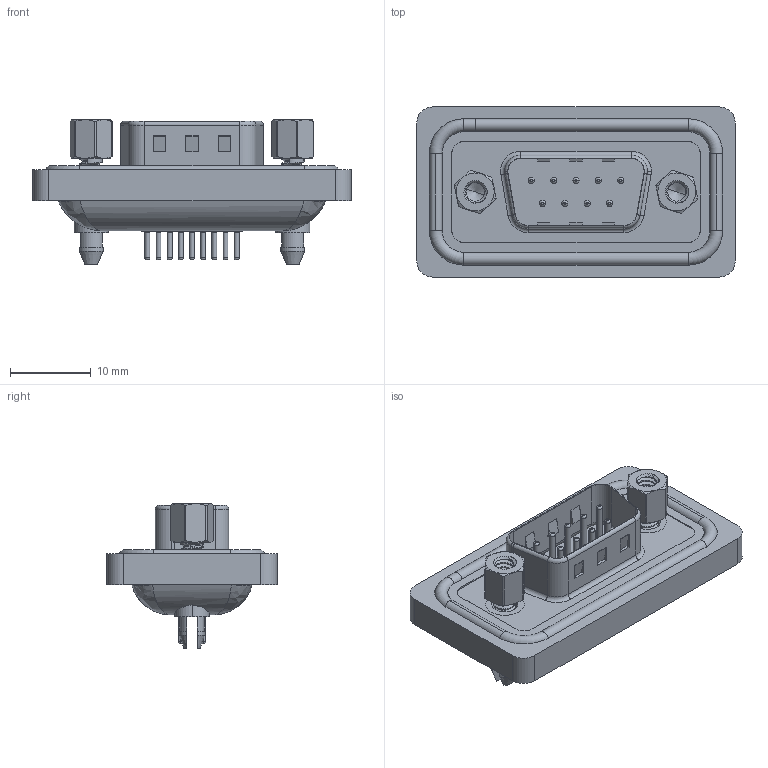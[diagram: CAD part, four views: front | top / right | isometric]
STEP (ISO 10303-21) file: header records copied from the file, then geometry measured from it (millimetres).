
FILE_DESCRIPTION (( 'STEP AP203' ), '1' );
FILE_NAME ('627-W09-320-013.STEP', '2024-03-19T11:55:11', ( '' ), ( '' ), 'SwSTEP 2.0', 'SolidWorks 2023', '' );
FILE_SCHEMA (( 'CONFIG_CONTROL_DESIGN' ));
Length unit declared in the file: millimetre
Products named in the file (8): 627W 4-40 Threaded Boardlock; 627W Contact Row 1_20; 627W Waterproof Housing_09 Contacts BL; 627W Housing_09 Contacts; 627W Contact Row 2_20; 627-W09-320-013; 627W 4-40 Hex Standoff; 627W Shell Front_09 Contacts
Assembly tree (16 placements, depth 2):
  627-W09-320-013
    627W Housing_09 Contacts
    627W Shell Front_09 Contacts
    627W Contact Row 1_20  x5
    627W Contact Row 2_20  x4
    627W Waterproof Housing_09 Contacts BL
    627W 4-40 Threaded Boardlock  x2
    627W 4-40 Hex Standoff  x2
Bounding box: 39.5 x 21.1 x 17.95 mm (x, y, z)
Volume: 4718.9 mm3; surface area: 6930.3 mm2
Topology: 17 solids, 17 shells, 847 faces, 2008 edges, 1251 vertices
Faces by surface type: cylinder 388, plane 218, torus 187, cone 32, bspline 22
Entity records: 20694 total; most frequent: CARTESIAN_POINT 7085, DIRECTION 2732, ORIENTED_EDGE 2574, EDGE_CURVE 1287, AXIS2_PLACEMENT_3D 1087, VERTEX_POINT 820, EDGE_LOOP 621, CIRCLE 559
